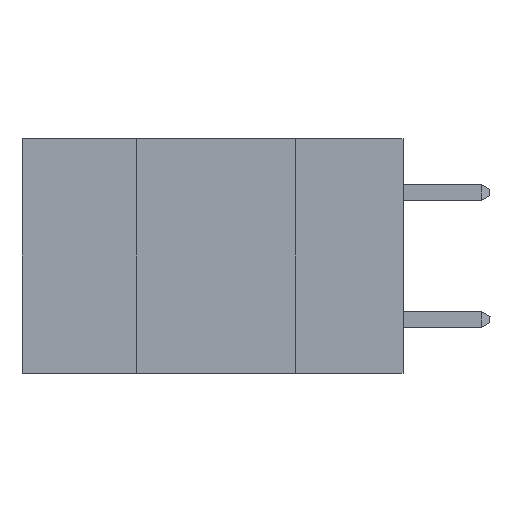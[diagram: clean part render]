
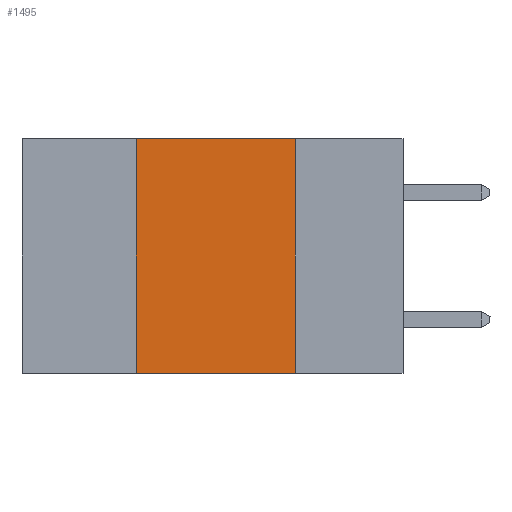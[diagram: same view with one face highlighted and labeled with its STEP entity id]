
A CAD part, left-side view. The second image highlights one B-rep face of the part: STEP entity #1495.
In plain terms, the highlighted planar face has unit normal (-1, 0, 0).
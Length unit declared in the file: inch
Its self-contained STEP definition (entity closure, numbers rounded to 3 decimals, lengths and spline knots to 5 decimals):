
#899 = VERTEX_POINT ( 'NONE', #16071 ) ;
#1495 = ADVANCED_FACE ( 'NONE', ( #3794 ), #4094, .F. ) ;
#2496 = VERTEX_POINT ( 'NONE', #29233 ) ;
#3794 = FACE_OUTER_BOUND ( 'NONE', #7391, .T. ) ;
#3948 = DIRECTION ( 'NONE',  ( 1., 0., 0. ) ) ;
#4094 = PLANE ( 'NONE',  #35697 ) ;
#4418 = LINE ( 'NONE', #8388, #30649 ) ;
#6203 = EDGE_CURVE ( 'NONE', #899, #2496, #31654, .T. ) ;
#6707 = EDGE_CURVE ( 'NONE', #8076, #2496, #7326, .T. ) ;
#7326 = LINE ( 'NONE', #37119, #26260 ) ;
#7391 = EDGE_LOOP ( 'NONE', ( #24391, #17858, #22097, #28245 ) ) ;
#8076 = VERTEX_POINT ( 'NONE', #41154 ) ;
#8388 = CARTESIAN_POINT ( 'NONE',  ( 0., 0.6, 0. ) ) ;
#9055 = EDGE_CURVE ( 'NONE', #8076, #20345, #30813, .T. ) ;
#10612 = EDGE_CURVE ( 'NONE', #20345, #899, #4418, .T. ) ;
#15833 = VECTOR ( 'NONE', #25396, 39.37008 ) ;
#16071 = CARTESIAN_POINT ( 'NONE',  ( 0., 0.17, 0. ) ) ;
#17594 = CARTESIAN_POINT ( 'NONE',  ( 0., 0.6, 0. ) ) ;
#17858 = ORIENTED_EDGE ( 'NONE', *, *, #10612, .F. ) ;
#20345 = VERTEX_POINT ( 'NONE', #20421 ) ;
#20421 = CARTESIAN_POINT ( 'NONE',  ( 0., 0.42, 0. ) ) ;
#20972 = DIRECTION ( 'NONE',  ( 0., 0., -1. ) ) ;
#22097 = ORIENTED_EDGE ( 'NONE', *, *, #9055, .F. ) ;
#22952 = DIRECTION ( 'NONE',  ( 0., 0., 1. ) ) ;
#24391 = ORIENTED_EDGE ( 'NONE', *, *, #6203, .F. ) ;
#25396 = DIRECTION ( 'NONE',  ( 0., 0., -1. ) ) ;
#26260 = VECTOR ( 'NONE', #37268, 39.37008 ) ;
#28245 = ORIENTED_EDGE ( 'NONE', *, *, #6707, .T. ) ;
#28705 = VECTOR ( 'NONE', #22952, 39.37008 ) ;
#29233 = CARTESIAN_POINT ( 'NONE',  ( 0., 0.17, -0.37 ) ) ;
#30649 = VECTOR ( 'NONE', #41942, 39.37008 ) ;
#30813 = LINE ( 'NONE', #33632, #28705 ) ;
#31654 = LINE ( 'NONE', #38325, #15833 ) ;
#33632 = CARTESIAN_POINT ( 'NONE',  ( 0., 0.42, 0. ) ) ;
#35697 = AXIS2_PLACEMENT_3D ( 'NONE', #17594, #3948, #20972 ) ;
#37119 = CARTESIAN_POINT ( 'NONE',  ( 0., 0.6, -0.37 ) ) ;
#37268 = DIRECTION ( 'NONE',  ( 0., -1., 0. ) ) ;
#38325 = CARTESIAN_POINT ( 'NONE',  ( 0., 0.17, 0. ) ) ;
#41154 = CARTESIAN_POINT ( 'NONE',  ( 0., 0.42, -0.37 ) ) ;
#41942 = DIRECTION ( 'NONE',  ( 0., -1., 0. ) ) ;
